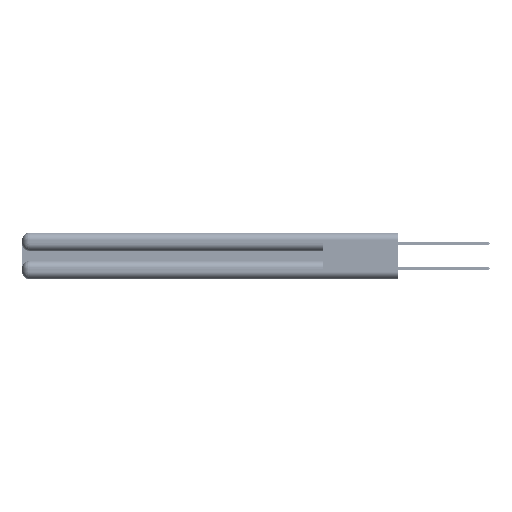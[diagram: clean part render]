
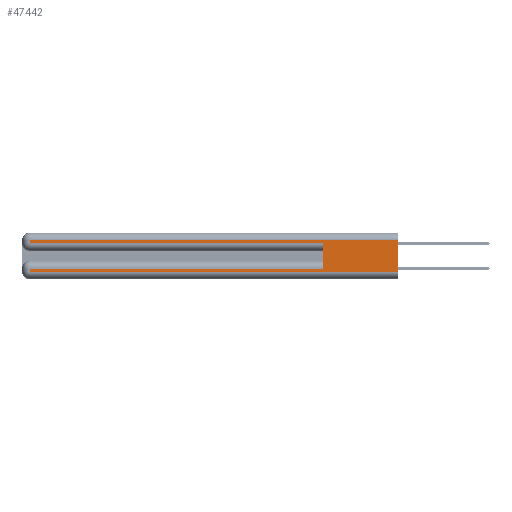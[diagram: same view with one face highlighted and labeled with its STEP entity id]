
A CAD part, left-side view. The second image highlights one B-rep face of the part: STEP entity #47442.
In plain terms, the highlighted planar face has unit normal (-1, 0, 0).
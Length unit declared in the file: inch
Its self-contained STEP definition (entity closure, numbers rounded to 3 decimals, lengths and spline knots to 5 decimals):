
#307 = CARTESIAN_POINT ( 'NONE',  ( 0., 2.94, 0.085 ) ) ;
#851 = FACE_OUTER_BOUND ( 'NONE', #44624, .T. ) ;
#2088 = CARTESIAN_POINT ( 'NONE',  ( 0., 0.6, 0.285 ) ) ;
#2115 = EDGE_CURVE ( 'NONE', #20672, #39233, #35633, .T. ) ;
#3931 = VECTOR ( 'NONE', #33122, 39.37008 ) ;
#4076 = ORIENTED_EDGE ( 'NONE', *, *, #2115, .F. ) ;
#4828 = CARTESIAN_POINT ( 'NONE',  ( 0., 2.94, 0.37 ) ) ;
#6592 = VERTEX_POINT ( 'NONE', #20492 ) ;
#6876 = VECTOR ( 'NONE', #51273, 39.37008 ) ;
#7025 = EDGE_CURVE ( 'NONE', #12881, #6592, #33422, .T. ) ;
#7497 = CARTESIAN_POINT ( 'NONE',  ( 0., 0., 0.37 ) ) ;
#7553 = VECTOR ( 'NONE', #13335, 39.37008 ) ;
#8865 = VECTOR ( 'NONE', #23664, 39.37008 ) ;
#10035 = EDGE_CURVE ( 'NONE', #6592, #39233, #23453, .T. ) ;
#11108 = VERTEX_POINT ( 'NONE', #45516 ) ;
#11130 = CARTESIAN_POINT ( 'NONE',  ( 0., 0., 0.37 ) ) ;
#11570 = PLANE ( 'NONE',  #52054 ) ;
#11705 = ORIENTED_EDGE ( 'NONE', *, *, #7025, .T. ) ;
#12721 = ORIENTED_EDGE ( 'NONE', *, *, #10035, .T. ) ;
#12804 = VERTEX_POINT ( 'NONE', #34448 ) ;
#12881 = VERTEX_POINT ( 'NONE', #307 ) ;
#13335 = DIRECTION ( 'NONE',  ( 0., 0., 1. ) ) ;
#14474 = DIRECTION ( 'NONE',  ( 0., 1., 0. ) ) ;
#14719 = ORIENTED_EDGE ( 'NONE', *, *, #25143, .T. ) ;
#15040 = VECTOR ( 'NONE', #57033, 39.37008 ) ;
#16073 = DIRECTION ( 'NONE',  ( 0., 1., 0. ) ) ;
#16194 = VERTEX_POINT ( 'NONE', #2088 ) ;
#16782 = DIRECTION ( 'NONE',  ( 0., 0., -1. ) ) ;
#18789 = VECTOR ( 'NONE', #16073, 39.37008 ) ;
#18866 = ORIENTED_EDGE ( 'NONE', *, *, #29494, .F. ) ;
#19310 = LINE ( 'NONE', #31446, #7553 ) ;
#20492 = CARTESIAN_POINT ( 'NONE',  ( 0., 2.94, 0.06 ) ) ;
#20672 = VERTEX_POINT ( 'NONE', #27510 ) ;
#21062 = CARTESIAN_POINT ( 'NONE',  ( 0., 0., 0.085 ) ) ;
#21995 = LINE ( 'NONE', #50050, #8865 ) ;
#23453 = LINE ( 'NONE', #25254, #6876 ) ;
#23664 = DIRECTION ( 'NONE',  ( 0., 0., -1. ) ) ;
#25021 = CARTESIAN_POINT ( 'NONE',  ( 0., 0., 0.06 ) ) ;
#25143 = EDGE_CURVE ( 'NONE', #20672, #11108, #53096, .T. ) ;
#25254 = CARTESIAN_POINT ( 'NONE',  ( 0., 0., 0.06 ) ) ;
#27510 = CARTESIAN_POINT ( 'NONE',  ( 0., 0., 0.31 ) ) ;
#28167 = VERTEX_POINT ( 'NONE', #42909 ) ;
#29494 = EDGE_CURVE ( 'NONE', #12804, #16194, #19310, .T. ) ;
#30328 = EDGE_CURVE ( 'NONE', #28167, #16194, #47410, .T. ) ;
#31446 = CARTESIAN_POINT ( 'NONE',  ( 0., 0.6, 0.145 ) ) ;
#33122 = DIRECTION ( 'NONE',  ( 0., 0., -1. ) ) ;
#33422 = LINE ( 'NONE', #4828, #53345 ) ;
#33820 = VECTOR ( 'NONE', #14474, 39.37008 ) ;
#34230 = ORIENTED_EDGE ( 'NONE', *, *, #30328, .T. ) ;
#34448 = CARTESIAN_POINT ( 'NONE',  ( 0., 0.6, 0.085 ) ) ;
#35242 = CARTESIAN_POINT ( 'NONE',  ( 0., 0., 0.285 ) ) ;
#35633 = LINE ( 'NONE', #11130, #3931 ) ;
#39233 = VERTEX_POINT ( 'NONE', #25021 ) ;
#40405 = EDGE_CURVE ( 'NONE', #12804, #12881, #48401, .T. ) ;
#40635 = DIRECTION ( 'NONE',  ( 0., 0., -1. ) ) ;
#42746 = DIRECTION ( 'NONE',  ( 1., 0., 0. ) ) ;
#42909 = CARTESIAN_POINT ( 'NONE',  ( 0., 2.94, 0.285 ) ) ;
#44624 = EDGE_LOOP ( 'NONE', ( #4076, #14719, #47222, #34230, #18866, #53143, #11705, #12721 ) ) ;
#45516 = CARTESIAN_POINT ( 'NONE',  ( 0., 2.94, 0.31 ) ) ;
#47222 = ORIENTED_EDGE ( 'NONE', *, *, #52590, .T. ) ;
#47410 = LINE ( 'NONE', #35242, #15040 ) ;
#47442 = ADVANCED_FACE ( 'NONE', ( #851 ), #11570, .F. ) ;
#48401 = LINE ( 'NONE', #21062, #18789 ) ;
#50050 = CARTESIAN_POINT ( 'NONE',  ( 0., 2.94, 0.37 ) ) ;
#51273 = DIRECTION ( 'NONE',  ( 0., -1., 0. ) ) ;
#52054 = AXIS2_PLACEMENT_3D ( 'NONE', #7497, #42746, #16782 ) ;
#52590 = EDGE_CURVE ( 'NONE', #11108, #28167, #21995, .T. ) ;
#53096 = LINE ( 'NONE', #54342, #33820 ) ;
#53143 = ORIENTED_EDGE ( 'NONE', *, *, #40405, .T. ) ;
#53345 = VECTOR ( 'NONE', #40635, 39.37008 ) ;
#54342 = CARTESIAN_POINT ( 'NONE',  ( 0., 0., 0.31 ) ) ;
#57033 = DIRECTION ( 'NONE',  ( 0., -1., 0. ) ) ;
